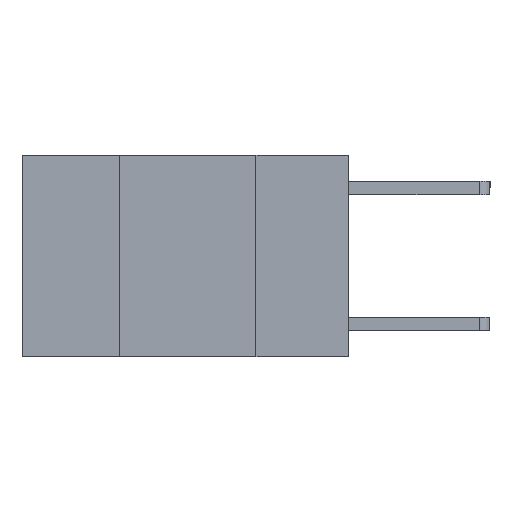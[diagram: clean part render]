
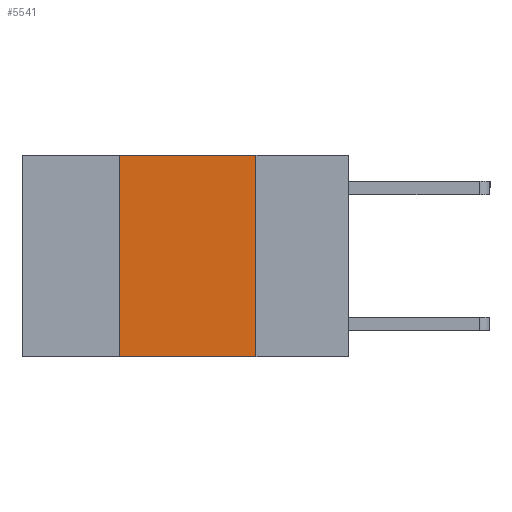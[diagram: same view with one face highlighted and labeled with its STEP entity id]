
A CAD part, left-side view. The second image highlights one B-rep face of the part: STEP entity #5541.
In plain terms, the highlighted planar face has unit normal (-1, 0, 0).
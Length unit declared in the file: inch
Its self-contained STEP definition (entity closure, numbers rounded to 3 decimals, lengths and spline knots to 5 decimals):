
#1364 = CARTESIAN_POINT ( 'NONE',  ( 0., 0.42, 0. ) ) ;
#1385 = DIRECTION ( 'NONE',  ( 1., 0., 0. ) ) ;
#1604 = EDGE_LOOP ( 'NONE', ( #4488, #8995, #11022, #9106 ) ) ;
#1846 = DIRECTION ( 'NONE',  ( 0., -1., 0. ) ) ;
#2197 = VERTEX_POINT ( 'NONE', #7139 ) ;
#2385 = DIRECTION ( 'NONE',  ( 0., 0., 1. ) ) ;
#3106 = VECTOR ( 'NONE', #6691, 39.37008 ) ;
#3124 = LINE ( 'NONE', #4958, #3106 ) ;
#3285 = VECTOR ( 'NONE', #1846, 39.37008 ) ;
#3459 = AXIS2_PLACEMENT_3D ( 'NONE', #8590, #1385, #10325 ) ;
#3572 = LINE ( 'NONE', #4318, #9178 ) ;
#4318 = CARTESIAN_POINT ( 'NONE',  ( 0., 0.17, 0. ) ) ;
#4488 = ORIENTED_EDGE ( 'NONE', *, *, #5790, .F. ) ;
#4574 = CARTESIAN_POINT ( 'NONE',  ( 0., 0.42, -0.37 ) ) ;
#4854 = VERTEX_POINT ( 'NONE', #4574 ) ;
#4958 = CARTESIAN_POINT ( 'NONE',  ( 0., 0.6, 0. ) ) ;
#5537 = EDGE_CURVE ( 'NONE', #9351, #2197, #3124, .T. ) ;
#5541 = ADVANCED_FACE ( 'NONE', ( #5937 ), #8475, .F. ) ;
#5706 = EDGE_CURVE ( 'NONE', #4854, #6956, #6047, .T. ) ;
#5790 = EDGE_CURVE ( 'NONE', #2197, #6956, #3572, .T. ) ;
#5892 = CARTESIAN_POINT ( 'NONE',  ( 0., 0.42, 0. ) ) ;
#5937 = FACE_OUTER_BOUND ( 'NONE', #1604, .T. ) ;
#6047 = LINE ( 'NONE', #7952, #3285 ) ;
#6691 = DIRECTION ( 'NONE',  ( 0., -1., 0. ) ) ;
#6956 = VERTEX_POINT ( 'NONE', #11329 ) ;
#7139 = CARTESIAN_POINT ( 'NONE',  ( 0., 0.17, 0. ) ) ;
#7140 = DIRECTION ( 'NONE',  ( 0., 0., -1. ) ) ;
#7952 = CARTESIAN_POINT ( 'NONE',  ( 0., 0.6, -0.37 ) ) ;
#8323 = VECTOR ( 'NONE', #2385, 39.37008 ) ;
#8475 = PLANE ( 'NONE',  #3459 ) ;
#8590 = CARTESIAN_POINT ( 'NONE',  ( 0., 0.6, 0. ) ) ;
#8995 = ORIENTED_EDGE ( 'NONE', *, *, #5537, .F. ) ;
#9106 = ORIENTED_EDGE ( 'NONE', *, *, #5706, .T. ) ;
#9178 = VECTOR ( 'NONE', #7140, 39.37008 ) ;
#9351 = VERTEX_POINT ( 'NONE', #1364 ) ;
#10325 = DIRECTION ( 'NONE',  ( 0., 0., -1. ) ) ;
#11022 = ORIENTED_EDGE ( 'NONE', *, *, #11144, .F. ) ;
#11144 = EDGE_CURVE ( 'NONE', #4854, #9351, #11342, .T. ) ;
#11329 = CARTESIAN_POINT ( 'NONE',  ( 0., 0.17, -0.37 ) ) ;
#11342 = LINE ( 'NONE', #5892, #8323 ) ;
